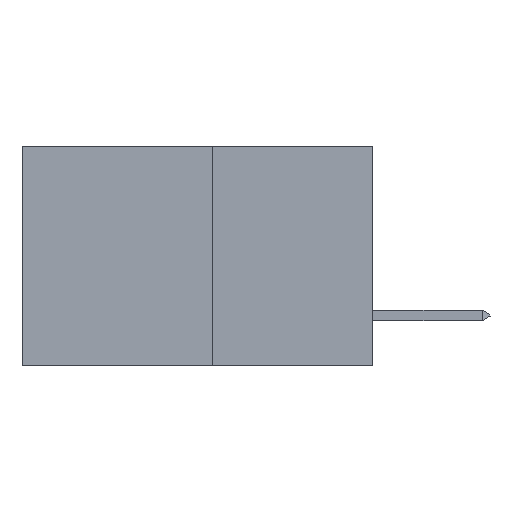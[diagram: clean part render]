
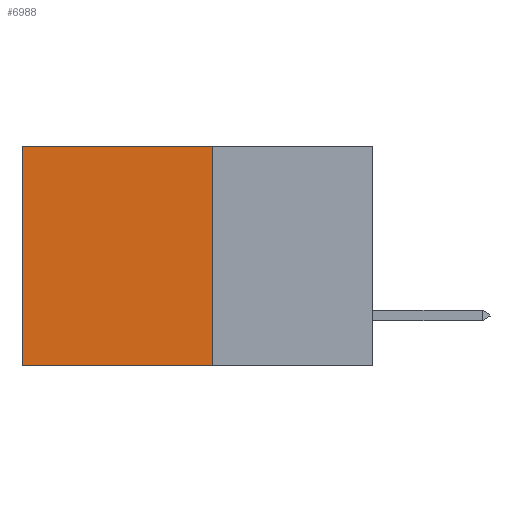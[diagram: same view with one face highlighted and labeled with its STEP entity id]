
A CAD part, left-side view. The second image highlights one B-rep face of the part: STEP entity #6988.
In plain terms, the highlighted planar face has unit normal (-1, 0, 0).
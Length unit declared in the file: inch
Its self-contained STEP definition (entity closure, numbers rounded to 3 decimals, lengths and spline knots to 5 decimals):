
#165 = CARTESIAN_POINT ( 'NONE',  ( 0.277, 0.27, -0.37 ) ) ;
#299 = FACE_OUTER_BOUND ( 'NONE', #3280, .T. ) ;
#483 = LINE ( 'NONE', #4007, #11902 ) ;
#719 = EDGE_CURVE ( 'NONE', #5776, #1143, #483, .T. ) ;
#1143 = VERTEX_POINT ( 'NONE', #8122 ) ;
#1491 = CARTESIAN_POINT ( 'NONE',  ( 0.277, 0.59, 0. ) ) ;
#1803 = EDGE_CURVE ( 'NONE', #4308, #5776, #5504, .T. ) ;
#1817 = VECTOR ( 'NONE', #12928, 39.37008 ) ;
#2202 = VECTOR ( 'NONE', #9286, 39.37008 ) ;
#2207 = EDGE_CURVE ( 'NONE', #4818, #1143, #10286, .T. ) ;
#2336 = CARTESIAN_POINT ( 'NONE',  ( 0.277, 0.27, -0.37 ) ) ;
#2400 = CARTESIAN_POINT ( 'NONE',  ( 0.277, 0.27, 0. ) ) ;
#3168 = ORIENTED_EDGE ( 'NONE', *, *, #5875, .T. ) ;
#3280 = EDGE_LOOP ( 'NONE', ( #4177, #11040, #11999, #3168 ) ) ;
#3529 = CARTESIAN_POINT ( 'NONE',  ( 0.277, 0.59, -0.37 ) ) ;
#4007 = CARTESIAN_POINT ( 'NONE',  ( 0.277, 0.27, -0.37 ) ) ;
#4177 = ORIENTED_EDGE ( 'NONE', *, *, #2207, .T. ) ;
#4308 = VERTEX_POINT ( 'NONE', #2400 ) ;
#4818 = VERTEX_POINT ( 'NONE', #1491 ) ;
#4846 = PLANE ( 'NONE',  #9491 ) ;
#5504 = LINE ( 'NONE', #10283, #1817 ) ;
#5776 = VERTEX_POINT ( 'NONE', #165 ) ;
#5875 = EDGE_CURVE ( 'NONE', #4308, #4818, #7083, .T. ) ;
#6988 = ADVANCED_FACE ( 'NONE', ( #299 ), #4846, .F. ) ;
#7083 = LINE ( 'NONE', #8657, #12067 ) ;
#8122 = CARTESIAN_POINT ( 'NONE',  ( 0.277, 0.59, -0.37 ) ) ;
#8152 = DIRECTION ( 'NONE',  ( 0., 0., -1. ) ) ;
#8657 = CARTESIAN_POINT ( 'NONE',  ( 0.277, 0.27, 0. ) ) ;
#9286 = DIRECTION ( 'NONE',  ( 0., 0., -1. ) ) ;
#9491 = AXIS2_PLACEMENT_3D ( 'NONE', #2336, #14022, #8152 ) ;
#10283 = CARTESIAN_POINT ( 'NONE',  ( 0.277, 0.27, -0.37 ) ) ;
#10286 = LINE ( 'NONE', #3529, #2202 ) ;
#10597 = DIRECTION ( 'NONE',  ( 0., 1., 0. ) ) ;
#11040 = ORIENTED_EDGE ( 'NONE', *, *, #719, .F. ) ;
#11237 = DIRECTION ( 'NONE',  ( 0., 1., 0. ) ) ;
#11902 = VECTOR ( 'NONE', #11237, 39.37008 ) ;
#11999 = ORIENTED_EDGE ( 'NONE', *, *, #1803, .F. ) ;
#12067 = VECTOR ( 'NONE', #10597, 39.37008 ) ;
#12928 = DIRECTION ( 'NONE',  ( 0., 0., -1. ) ) ;
#14022 = DIRECTION ( 'NONE',  ( 1., 0., 0. ) ) ;
